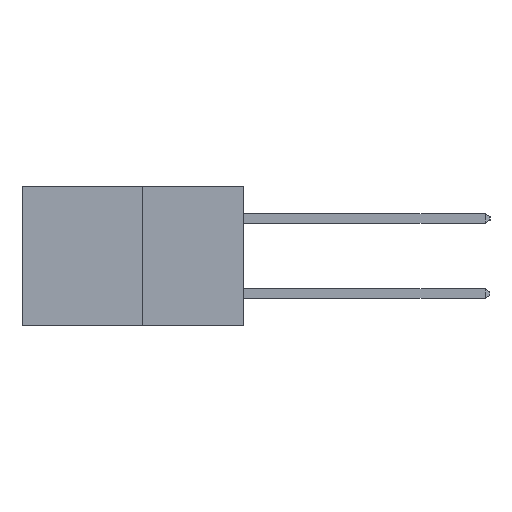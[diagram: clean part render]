
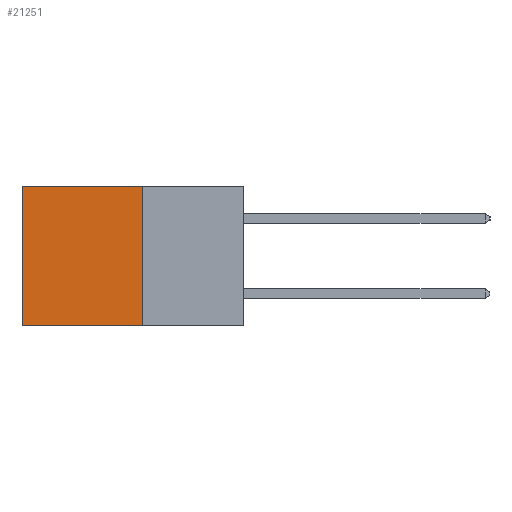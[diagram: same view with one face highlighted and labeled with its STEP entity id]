
A CAD part, left-side view. The second image highlights one B-rep face of the part: STEP entity #21251.
In plain terms, the highlighted planar face has unit normal (-1, 0, 0).
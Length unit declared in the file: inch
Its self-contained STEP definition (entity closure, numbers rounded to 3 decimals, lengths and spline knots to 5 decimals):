
#1784 = DIRECTION ( 'NONE',  ( 0., 0., -1. ) ) ;
#1895 = EDGE_LOOP ( 'NONE', ( #17765, #8745, #25515, #3882 ) ) ;
#2862 = EDGE_CURVE ( 'NONE', #24181, #25835, #24976, .T. ) ;
#3045 = EDGE_CURVE ( 'NONE', #7078, #25835, #26085, .T. ) ;
#3515 = DIRECTION ( 'NONE',  ( 0., 1., 0. ) ) ;
#3684 = CARTESIAN_POINT ( 'NONE',  ( 0.277, 0.27, -0.37 ) ) ;
#3882 = ORIENTED_EDGE ( 'NONE', *, *, #15015, .T. ) ;
#5003 = CARTESIAN_POINT ( 'NONE',  ( 0.277, 0.27, 0. ) ) ;
#6104 = VECTOR ( 'NONE', #18064, 39.37008 ) ;
#6109 = VECTOR ( 'NONE', #1784, 39.37008 ) ;
#6857 = LINE ( 'NONE', #15601, #6104 ) ;
#7078 = VERTEX_POINT ( 'NONE', #24561 ) ;
#8090 = DIRECTION ( 'NONE',  ( 1., 0., 0. ) ) ;
#8745 = ORIENTED_EDGE ( 'NONE', *, *, #2862, .F. ) ;
#13429 = CARTESIAN_POINT ( 'NONE',  ( 0.277, 0.59, -0.37 ) ) ;
#15015 = EDGE_CURVE ( 'NONE', #21215, #7078, #6857, .T. ) ;
#15601 = CARTESIAN_POINT ( 'NONE',  ( 0.277, 0.27, 0. ) ) ;
#17250 = VECTOR ( 'NONE', #23491, 39.37008 ) ;
#17734 = PLANE ( 'NONE',  #20020 ) ;
#17765 = ORIENTED_EDGE ( 'NONE', *, *, #3045, .T. ) ;
#18064 = DIRECTION ( 'NONE',  ( 0., 1., 0. ) ) ;
#18782 = CARTESIAN_POINT ( 'NONE',  ( 0.277, 0.59, -0.37 ) ) ;
#20020 = AXIS2_PLACEMENT_3D ( 'NONE', #22563, #8090, #24945 ) ;
#21096 = CARTESIAN_POINT ( 'NONE',  ( 0.277, 0.27, -0.37 ) ) ;
#21215 = VERTEX_POINT ( 'NONE', #5003 ) ;
#21251 = ADVANCED_FACE ( 'NONE', ( #26983 ), #17734, .F. ) ;
#22563 = CARTESIAN_POINT ( 'NONE',  ( 0.277, 0.27, -0.37 ) ) ;
#22874 = CARTESIAN_POINT ( 'NONE',  ( 0.277, 0.27, -0.37 ) ) ;
#23491 = DIRECTION ( 'NONE',  ( 0., 0., -1. ) ) ;
#24181 = VERTEX_POINT ( 'NONE', #3684 ) ;
#24561 = CARTESIAN_POINT ( 'NONE',  ( 0.277, 0.59, 0. ) ) ;
#24945 = DIRECTION ( 'NONE',  ( 0., 0., -1. ) ) ;
#24976 = LINE ( 'NONE', #22874, #30563 ) ;
#25515 = ORIENTED_EDGE ( 'NONE', *, *, #29280, .F. ) ;
#25835 = VERTEX_POINT ( 'NONE', #13429 ) ;
#26085 = LINE ( 'NONE', #18782, #6109 ) ;
#26983 = FACE_OUTER_BOUND ( 'NONE', #1895, .T. ) ;
#29280 = EDGE_CURVE ( 'NONE', #21215, #24181, #29965, .T. ) ;
#29965 = LINE ( 'NONE', #21096, #17250 ) ;
#30563 = VECTOR ( 'NONE', #3515, 39.37008 ) ;
